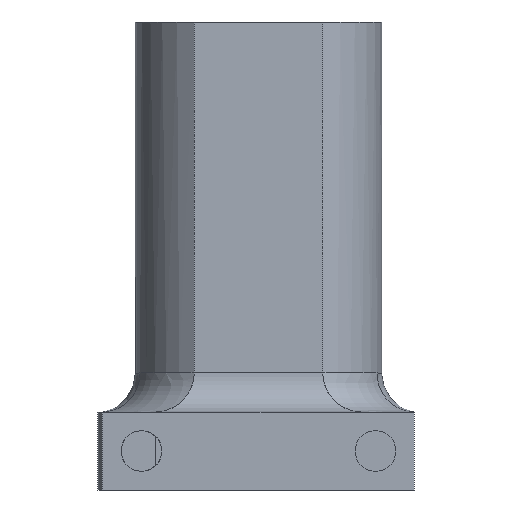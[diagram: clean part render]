
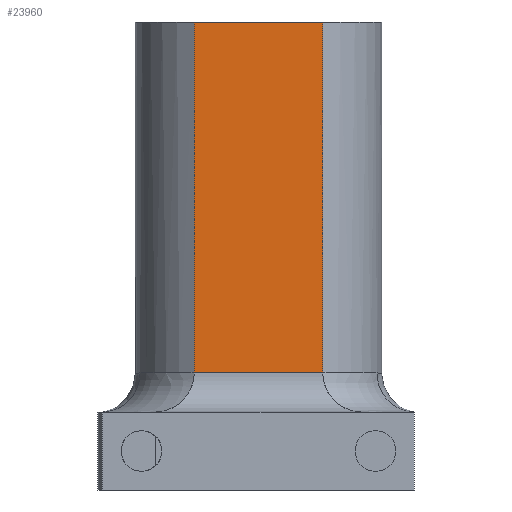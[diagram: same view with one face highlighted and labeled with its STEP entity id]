
A CAD part, front view. The second image highlights one B-rep face of the part: STEP entity #23960.
In plain terms, the highlighted planar face has unit normal (0, -1, 0).
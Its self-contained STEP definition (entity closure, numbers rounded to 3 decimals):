
#7764 = PLANE('',#7765);
#7765 = AXIS2_PLACEMENT_3D('',#7766,#7767,#7768);
#7766 = CARTESIAN_POINT('',(10.478,12.336,12.7));
#7767 = DIRECTION('',(-1.,0.,0.));
#7768 = DIRECTION('',(0.,1.,0.));
#7793 = PLANE('',#7794);
#7794 = AXIS2_PLACEMENT_3D('',#7795,#7796,#7797);
#7795 = CARTESIAN_POINT('',(-10.478,20.972,76.2));
#7796 = DIRECTION('',(0.,0.,-1.));
#7797 = DIRECTION('',(-1.,0.,0.));
#7825 = PLANE('',#7826);
#7826 = AXIS2_PLACEMENT_3D('',#7827,#7828,#7829);
#7827 = CARTESIAN_POINT('',(-10.478,20.972,12.7));
#7828 = DIRECTION('',(1.,0.,0.));
#7829 = DIRECTION('',(0.,-1.,0.));
#19621 = EDGE_CURVE('',#19622,#19624,#19626,.T.);
#19622 = VERTEX_POINT('',#19623);
#19623 = CARTESIAN_POINT('',(10.478,12.336,19.05));
#19624 = VERTEX_POINT('',#19625);
#19625 = CARTESIAN_POINT('',(10.478,12.336,76.2));
#19626 = SURFACE_CURVE('',#19627,(#19631,#19638),.PCURVE_S1.);
#19627 = LINE('',#19628,#19629);
#19628 = CARTESIAN_POINT('',(10.478,12.336,12.7));
#19629 = VECTOR('',#19630,1.);
#19630 = DIRECTION('',(0.,0.,1.));
#19631 = PCURVE('',#7764,#19632);
#19632 = DEFINITIONAL_REPRESENTATION('',(#19633),#19637);
#19633 = LINE('',#19634,#19635);
#19634 = CARTESIAN_POINT('',(0.,0.));
#19635 = VECTOR('',#19636,1.);
#19636 = DIRECTION('',(0.,-1.));
#19637 = ( GEOMETRIC_REPRESENTATION_CONTEXT(2) 
PARAMETRIC_REPRESENTATION_CONTEXT() REPRESENTATION_CONTEXT('2D SPACE',''
  ) );
#19638 = PCURVE('',#19639,#19644);
#19639 = PLANE('',#19640);
#19640 = AXIS2_PLACEMENT_3D('',#19641,#19642,#19643);
#19641 = CARTESIAN_POINT('',(-10.478,12.336,12.7));
#19642 = DIRECTION('',(0.,1.,0.));
#19643 = DIRECTION('',(1.,0.,0.));
#19644 = DEFINITIONAL_REPRESENTATION('',(#19645),#19649);
#19645 = LINE('',#19646,#19647);
#19646 = CARTESIAN_POINT('',(20.955,0.));
#19647 = VECTOR('',#19648,1.);
#19648 = DIRECTION('',(0.,-1.));
#19649 = ( GEOMETRIC_REPRESENTATION_CONTEXT(2) 
PARAMETRIC_REPRESENTATION_CONTEXT() REPRESENTATION_CONTEXT('2D SPACE',''
  ) );
#20073 = VERTEX_POINT('',#20074);
#20074 = CARTESIAN_POINT('',(-10.478,12.336,76.2));
#20095 = EDGE_CURVE('',#20073,#19624,#20096,.T.);
#20096 = SURFACE_CURVE('',#20097,(#20101,#20108),.PCURVE_S1.);
#20097 = LINE('',#20098,#20099);
#20098 = CARTESIAN_POINT('',(-10.478,12.336,76.2));
#20099 = VECTOR('',#20100,1.);
#20100 = DIRECTION('',(1.,0.,0.));
#20101 = PCURVE('',#7793,#20102);
#20102 = DEFINITIONAL_REPRESENTATION('',(#20103),#20107);
#20103 = LINE('',#20104,#20105);
#20104 = CARTESIAN_POINT('',(0.,-8.636));
#20105 = VECTOR('',#20106,1.);
#20106 = DIRECTION('',(-1.,0.));
#20107 = ( GEOMETRIC_REPRESENTATION_CONTEXT(2) 
PARAMETRIC_REPRESENTATION_CONTEXT() REPRESENTATION_CONTEXT('2D SPACE',''
  ) );
#20108 = PCURVE('',#19639,#20109);
#20109 = DEFINITIONAL_REPRESENTATION('',(#20110),#20114);
#20110 = LINE('',#20111,#20112);
#20111 = CARTESIAN_POINT('',(0.,-63.5));
#20112 = VECTOR('',#20113,1.);
#20113 = DIRECTION('',(1.,0.));
#20114 = ( GEOMETRIC_REPRESENTATION_CONTEXT(2) 
PARAMETRIC_REPRESENTATION_CONTEXT() REPRESENTATION_CONTEXT('2D SPACE',''
  ) );
#20242 = EDGE_CURVE('',#20243,#20073,#20245,.T.);
#20243 = VERTEX_POINT('',#20244);
#20244 = CARTESIAN_POINT('',(-10.478,12.336,19.05));
#20245 = SURFACE_CURVE('',#20246,(#20250,#20257),.PCURVE_S1.);
#20246 = LINE('',#20247,#20248);
#20247 = CARTESIAN_POINT('',(-10.478,12.336,12.7));
#20248 = VECTOR('',#20249,1.);
#20249 = DIRECTION('',(0.,0.,1.));
#20250 = PCURVE('',#7825,#20251);
#20251 = DEFINITIONAL_REPRESENTATION('',(#20252),#20256);
#20252 = LINE('',#20253,#20254);
#20253 = CARTESIAN_POINT('',(8.636,0.));
#20254 = VECTOR('',#20255,1.);
#20255 = DIRECTION('',(0.,-1.));
#20256 = ( GEOMETRIC_REPRESENTATION_CONTEXT(2) 
PARAMETRIC_REPRESENTATION_CONTEXT() REPRESENTATION_CONTEXT('2D SPACE',''
  ) );
#20257 = PCURVE('',#19639,#20258);
#20258 = DEFINITIONAL_REPRESENTATION('',(#20259),#20263);
#20259 = LINE('',#20260,#20261);
#20260 = CARTESIAN_POINT('',(0.,0.));
#20261 = VECTOR('',#20262,1.);
#20262 = DIRECTION('',(0.,-1.));
#20263 = ( GEOMETRIC_REPRESENTATION_CONTEXT(2) 
PARAMETRIC_REPRESENTATION_CONTEXT() REPRESENTATION_CONTEXT('2D SPACE',''
  ) );
#20710 = CYLINDRICAL_SURFACE('',#20711,6.35);
#20711 = AXIS2_PLACEMENT_3D('',#20712,#20713,#20714);
#20712 = CARTESIAN_POINT('',(-10.478,5.986,19.05));
#20713 = DIRECTION('',(1.,0.,0.));
#20714 = DIRECTION('',(0.,0.,-1.));
#23960 = ADVANCED_FACE('',(#23961),#19639,.F.);
#23961 = FACE_BOUND('',#23962,.F.);
#23962 = EDGE_LOOP('',(#23963,#23964,#23965,#23966));
#23963 = ORIENTED_EDGE('',*,*,#20242,.T.);
#23964 = ORIENTED_EDGE('',*,*,#20095,.T.);
#23965 = ORIENTED_EDGE('',*,*,#19621,.F.);
#23966 = ORIENTED_EDGE('',*,*,#23967,.F.);
#23967 = EDGE_CURVE('',#20243,#19622,#23968,.T.);
#23968 = SURFACE_CURVE('',#23969,(#23973,#23980),.PCURVE_S1.);
#23969 = LINE('',#23970,#23971);
#23970 = CARTESIAN_POINT('',(-10.478,12.336,19.05));
#23971 = VECTOR('',#23972,1.);
#23972 = DIRECTION('',(1.,0.,0.));
#23973 = PCURVE('',#19639,#23974);
#23974 = DEFINITIONAL_REPRESENTATION('',(#23975),#23979);
#23975 = LINE('',#23976,#23977);
#23976 = CARTESIAN_POINT('',(0.,-6.35));
#23977 = VECTOR('',#23978,1.);
#23978 = DIRECTION('',(1.,0.));
#23979 = ( GEOMETRIC_REPRESENTATION_CONTEXT(2) 
PARAMETRIC_REPRESENTATION_CONTEXT() REPRESENTATION_CONTEXT('2D SPACE',''
  ) );
#23980 = PCURVE('',#20710,#23981);
#23981 = DEFINITIONAL_REPRESENTATION('',(#23982),#23986);
#23982 = LINE('',#23983,#23984);
#23983 = CARTESIAN_POINT('',(1.571,0.));
#23984 = VECTOR('',#23985,1.);
#23985 = DIRECTION('',(0.,1.));
#23986 = ( GEOMETRIC_REPRESENTATION_CONTEXT(2) 
PARAMETRIC_REPRESENTATION_CONTEXT() REPRESENTATION_CONTEXT('2D SPACE',''
  ) );
